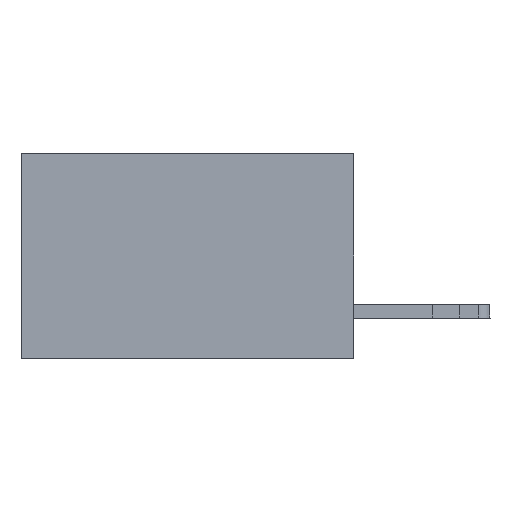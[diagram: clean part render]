
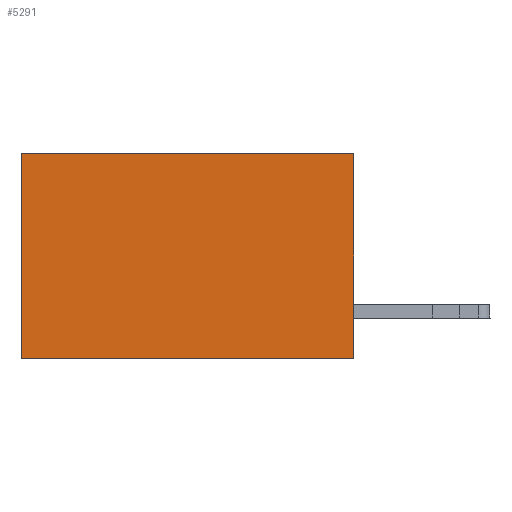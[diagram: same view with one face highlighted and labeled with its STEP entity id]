
A CAD part, left-side view. The second image highlights one B-rep face of the part: STEP entity #5291.
In plain terms, the highlighted planar face has unit normal (-1, 0, 0).
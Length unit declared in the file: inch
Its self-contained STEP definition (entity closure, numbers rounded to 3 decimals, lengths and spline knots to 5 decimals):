
#1535 = VECTOR ( 'NONE', #12098, 39.37008 ) ;
#2047 = EDGE_CURVE ( 'NONE', #16419, #17853, #18916, .T. ) ;
#2834 = ORIENTED_EDGE ( 'NONE', *, *, #14299, .T. ) ;
#3669 = ORIENTED_EDGE ( 'NONE', *, *, #21377, .T. ) ;
#4211 = EDGE_LOOP ( 'NONE', ( #3669, #10059, #19274, #2834 ) ) ;
#5291 = ADVANCED_FACE ( 'NONE', ( #20925 ), #7873, .F. ) ;
#5327 = VECTOR ( 'NONE', #17942, 39.37008 ) ;
#5564 = CARTESIAN_POINT ( 'NONE',  ( 0.2875, 0., 0. ) ) ;
#6688 = LINE ( 'NONE', #21340, #1535 ) ;
#7873 = PLANE ( 'NONE',  #17446 ) ;
#9556 = DIRECTION ( 'NONE',  ( 0., 0., -1. ) ) ;
#9673 = CARTESIAN_POINT ( 'NONE',  ( 0.2875, 0., -0.37 ) ) ;
#9906 = VECTOR ( 'NONE', #16960, 39.37008 ) ;
#10059 = ORIENTED_EDGE ( 'NONE', *, *, #11761, .F. ) ;
#10078 = DIRECTION ( 'NONE',  ( 0., 1., 0. ) ) ;
#11305 = DIRECTION ( 'NONE',  ( 1., 0., 0. ) ) ;
#11761 = EDGE_CURVE ( 'NONE', #17853, #21140, #6688, .T. ) ;
#12098 = DIRECTION ( 'NONE',  ( 0., 1., 0. ) ) ;
#14035 = LINE ( 'NONE', #17781, #5327 ) ;
#14299 = EDGE_CURVE ( 'NONE', #16419, #18199, #22050, .T. ) ;
#14358 = CARTESIAN_POINT ( 'NONE',  ( 0.2875, 0., 0. ) ) ;
#16296 = VECTOR ( 'NONE', #10078, 39.37008 ) ;
#16419 = VERTEX_POINT ( 'NONE', #14358 ) ;
#16960 = DIRECTION ( 'NONE',  ( 0., 0., -1. ) ) ;
#17194 = CARTESIAN_POINT ( 'NONE',  ( 0.2875, 0.6, 0. ) ) ;
#17446 = AXIS2_PLACEMENT_3D ( 'NONE', #20466, #11305, #9556 ) ;
#17781 = CARTESIAN_POINT ( 'NONE',  ( 0.2875, 0.6, 0. ) ) ;
#17853 = VERTEX_POINT ( 'NONE', #9673 ) ;
#17942 = DIRECTION ( 'NONE',  ( 0., 0., -1. ) ) ;
#18060 = CARTESIAN_POINT ( 'NONE',  ( 0.2875, 0.6, -0.37 ) ) ;
#18199 = VERTEX_POINT ( 'NONE', #17194 ) ;
#18916 = LINE ( 'NONE', #5564, #9906 ) ;
#19274 = ORIENTED_EDGE ( 'NONE', *, *, #2047, .F. ) ;
#20466 = CARTESIAN_POINT ( 'NONE',  ( 0.2875, 0., 0. ) ) ;
#20925 = FACE_OUTER_BOUND ( 'NONE', #4211, .T. ) ;
#21085 = CARTESIAN_POINT ( 'NONE',  ( 0.2875, 0., 0. ) ) ;
#21140 = VERTEX_POINT ( 'NONE', #18060 ) ;
#21340 = CARTESIAN_POINT ( 'NONE',  ( 0.2875, 0., -0.37 ) ) ;
#21377 = EDGE_CURVE ( 'NONE', #18199, #21140, #14035, .T. ) ;
#22050 = LINE ( 'NONE', #21085, #16296 ) ;
